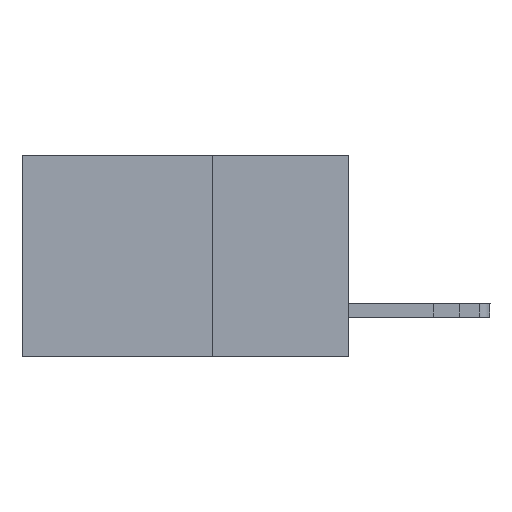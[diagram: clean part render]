
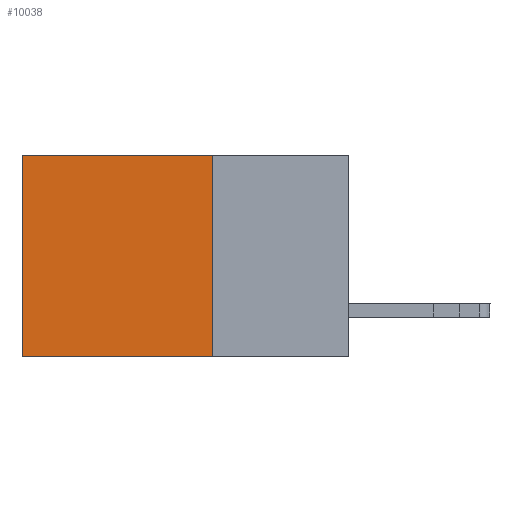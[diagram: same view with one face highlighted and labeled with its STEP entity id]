
A CAD part, left-side view. The second image highlights one B-rep face of the part: STEP entity #10038.
In plain terms, the highlighted planar face has unit normal (-1, 0, 0).
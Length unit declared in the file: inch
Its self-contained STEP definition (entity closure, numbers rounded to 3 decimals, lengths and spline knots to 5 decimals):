
#336 = EDGE_CURVE ( 'NONE', #10529, #7964, #6525, .T. ) ;
#484 = LINE ( 'NONE', #11283, #1434 ) ;
#1135 = CARTESIAN_POINT ( 'NONE',  ( 0.2615, 0.25, -0.37 ) ) ;
#1434 = VECTOR ( 'NONE', #1563, 39.37008 ) ;
#1563 = DIRECTION ( 'NONE',  ( 0., 0., -1. ) ) ;
#1605 = DIRECTION ( 'NONE',  ( 0., 0., -1. ) ) ;
#1994 = EDGE_CURVE ( 'NONE', #10104, #10798, #7241, .T. ) ;
#2126 = ORIENTED_EDGE ( 'NONE', *, *, #7401, .F. ) ;
#2484 = VECTOR ( 'NONE', #3412, 39.37008 ) ;
#2581 = CARTESIAN_POINT ( 'NONE',  ( 0.2615, 0.6, 0. ) ) ;
#3031 = CARTESIAN_POINT ( 'NONE',  ( 0.2615, 0.25, -0.37 ) ) ;
#3046 = ORIENTED_EDGE ( 'NONE', *, *, #11023, .T. ) ;
#3412 = DIRECTION ( 'NONE',  ( 0., 1., 0. ) ) ;
#3501 = CARTESIAN_POINT ( 'NONE',  ( 0.2615, 0.6, -0.37 ) ) ;
#5036 = FACE_OUTER_BOUND ( 'NONE', #5806, .T. ) ;
#5611 = DIRECTION ( 'NONE',  ( 0., 0., -1. ) ) ;
#5612 = CARTESIAN_POINT ( 'NONE',  ( 0.2615, 0.25, 0. ) ) ;
#5806 = EDGE_LOOP ( 'NONE', ( #3046, #9802, #2126, #6041 ) ) ;
#5939 = PLANE ( 'NONE',  #11860 ) ;
#6041 = ORIENTED_EDGE ( 'NONE', *, *, #336, .T. ) ;
#6141 = VECTOR ( 'NONE', #5611, 39.37008 ) ;
#6525 = LINE ( 'NONE', #5612, #2484 ) ;
#6594 = LINE ( 'NONE', #1135, #6141 ) ;
#7241 = LINE ( 'NONE', #11571, #10804 ) ;
#7269 = CARTESIAN_POINT ( 'NONE',  ( 0.2615, 0.25, 0. ) ) ;
#7401 = EDGE_CURVE ( 'NONE', #10529, #10104, #6594, .T. ) ;
#7964 = VERTEX_POINT ( 'NONE', #2581 ) ;
#9190 = DIRECTION ( 'NONE',  ( 1., 0., 0. ) ) ;
#9802 = ORIENTED_EDGE ( 'NONE', *, *, #1994, .F. ) ;
#10038 = ADVANCED_FACE ( 'NONE', ( #5036 ), #5939, .F. ) ;
#10104 = VERTEX_POINT ( 'NONE', #3031 ) ;
#10529 = VERTEX_POINT ( 'NONE', #7269 ) ;
#10798 = VERTEX_POINT ( 'NONE', #3501 ) ;
#10804 = VECTOR ( 'NONE', #13854, 39.37008 ) ;
#11023 = EDGE_CURVE ( 'NONE', #7964, #10798, #484, .T. ) ;
#11283 = CARTESIAN_POINT ( 'NONE',  ( 0.2615, 0.6, -0.37 ) ) ;
#11547 = CARTESIAN_POINT ( 'NONE',  ( 0.2615, 0.25, -0.37 ) ) ;
#11571 = CARTESIAN_POINT ( 'NONE',  ( 0.2615, 0.25, -0.37 ) ) ;
#11860 = AXIS2_PLACEMENT_3D ( 'NONE', #11547, #9190, #1605 ) ;
#13854 = DIRECTION ( 'NONE',  ( 0., 1., 0. ) ) ;
